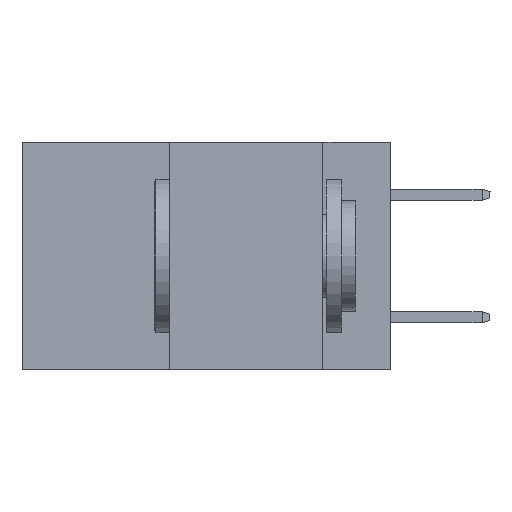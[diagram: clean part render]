
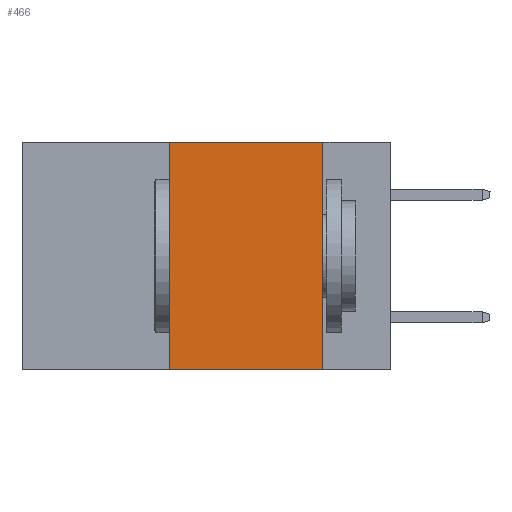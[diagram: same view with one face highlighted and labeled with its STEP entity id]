
A CAD part, left-side view. The second image highlights one B-rep face of the part: STEP entity #466.
In plain terms, the highlighted planar face has unit normal (-1, 0, 0).
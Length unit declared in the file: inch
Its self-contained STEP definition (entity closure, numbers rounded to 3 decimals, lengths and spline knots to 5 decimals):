
#466 = ADVANCED_FACE ( 'NONE', ( #5829 ), #14993, .F. ) ;
#2636 = VERTEX_POINT ( 'NONE', #13642 ) ;
#4150 = EDGE_CURVE ( 'NONE', #18701, #9280, #30133, .T. ) ;
#4163 = EDGE_LOOP ( 'NONE', ( #13670, #12778, #23411, #30023 ) ) ;
#5716 = DIRECTION ( 'NONE',  ( 0., -1., 0. ) ) ;
#5829 = FACE_OUTER_BOUND ( 'NONE', #4163, .T. ) ;
#7697 = CARTESIAN_POINT ( 'NONE',  ( 0., 0.6, 0. ) ) ;
#8418 = EDGE_CURVE ( 'NONE', #2636, #13591, #16775, .T. ) ;
#9280 = VERTEX_POINT ( 'NONE', #27190 ) ;
#10512 = DIRECTION ( 'NONE',  ( 0., 0., -1. ) ) ;
#10778 = CARTESIAN_POINT ( 'NONE',  ( 0., 0.6, 0. ) ) ;
#10839 = EDGE_CURVE ( 'NONE', #2636, #9280, #21434, .T. ) ;
#11508 = DIRECTION ( 'NONE',  ( 0., -1., 0. ) ) ;
#12012 = VECTOR ( 'NONE', #5716, 39.37008 ) ;
#12778 = ORIENTED_EDGE ( 'NONE', *, *, #21216, .F. ) ;
#13591 = VERTEX_POINT ( 'NONE', #20617 ) ;
#13642 = CARTESIAN_POINT ( 'NONE',  ( 0., 0.36, -0.37 ) ) ;
#13670 = ORIENTED_EDGE ( 'NONE', *, *, #4150, .F. ) ;
#14993 = PLANE ( 'NONE',  #18900 ) ;
#16775 = LINE ( 'NONE', #27490, #18649 ) ;
#18433 = DIRECTION ( 'NONE',  ( 0., 0., 1. ) ) ;
#18593 = CARTESIAN_POINT ( 'NONE',  ( 0., 0.6, -0.37 ) ) ;
#18649 = VECTOR ( 'NONE', #18433, 39.37008 ) ;
#18701 = VERTEX_POINT ( 'NONE', #24295 ) ;
#18900 = AXIS2_PLACEMENT_3D ( 'NONE', #7697, #20188, #10512 ) ;
#20188 = DIRECTION ( 'NONE',  ( 1., 0., 0. ) ) ;
#20617 = CARTESIAN_POINT ( 'NONE',  ( 0., 0.36, 0. ) ) ;
#21216 = EDGE_CURVE ( 'NONE', #13591, #18701, #28719, .T. ) ;
#21434 = LINE ( 'NONE', #18593, #28220 ) ;
#23411 = ORIENTED_EDGE ( 'NONE', *, *, #8418, .F. ) ;
#24295 = CARTESIAN_POINT ( 'NONE',  ( 0., 0.11, 0. ) ) ;
#26120 = DIRECTION ( 'NONE',  ( 0., 0., -1. ) ) ;
#27190 = CARTESIAN_POINT ( 'NONE',  ( 0., 0.11, -0.37 ) ) ;
#27490 = CARTESIAN_POINT ( 'NONE',  ( 0., 0.36, 0. ) ) ;
#28220 = VECTOR ( 'NONE', #11508, 39.37008 ) ;
#28641 = VECTOR ( 'NONE', #26120, 39.37008 ) ;
#28719 = LINE ( 'NONE', #10778, #12012 ) ;
#30023 = ORIENTED_EDGE ( 'NONE', *, *, #10839, .T. ) ;
#30133 = LINE ( 'NONE', #30530, #28641 ) ;
#30530 = CARTESIAN_POINT ( 'NONE',  ( 0., 0.11, 0. ) ) ;
